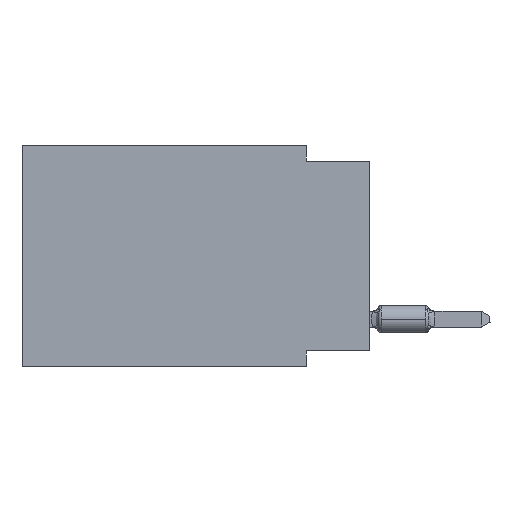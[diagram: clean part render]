
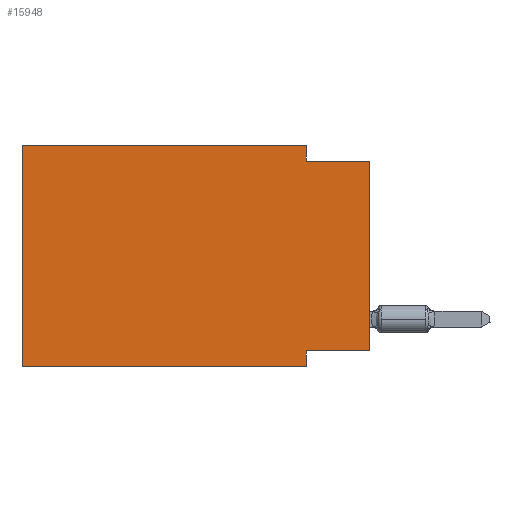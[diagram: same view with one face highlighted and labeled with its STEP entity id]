
A CAD part, left-side view. The second image highlights one B-rep face of the part: STEP entity #15948.
In plain terms, the highlighted planar face has unit normal (-1, 0, 0).
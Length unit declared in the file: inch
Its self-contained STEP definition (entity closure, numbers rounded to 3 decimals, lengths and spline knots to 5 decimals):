
#21 = VERTEX_POINT ( 'NONE', #21464 ) ;
#82 = PLANE ( 'NONE',  #12504 ) ;
#561 = ORIENTED_EDGE ( 'NONE', *, *, #11492, .F. ) ;
#1091 = DIRECTION ( 'NONE',  ( 0., -1., 0. ) ) ;
#1288 = VECTOR ( 'NONE', #1091, 39.37008 ) ;
#1444 = CARTESIAN_POINT ( 'NONE',  ( 0., 0.55, -0.35 ) ) ;
#1791 = LINE ( 'NONE', #2118, #21281 ) ;
#1793 = VECTOR ( 'NONE', #25685, 39.37008 ) ;
#2018 = CARTESIAN_POINT ( 'NONE',  ( 0., 0.1, 0. ) ) ;
#2118 = CARTESIAN_POINT ( 'NONE',  ( 0., 0., -0.325 ) ) ;
#2986 = VERTEX_POINT ( 'NONE', #25995 ) ;
#3607 = ORIENTED_EDGE ( 'NONE', *, *, #14719, .F. ) ;
#3935 = LINE ( 'NONE', #24307, #24319 ) ;
#4313 = VECTOR ( 'NONE', #11893, 39.37008 ) ;
#4394 = CARTESIAN_POINT ( 'NONE',  ( 0., 0.1, -0.35 ) ) ;
#4684 = LINE ( 'NONE', #2018, #8402 ) ;
#4748 = FACE_OUTER_BOUND ( 'NONE', #13828, .T. ) ;
#6435 = DIRECTION ( 'NONE',  ( 0., -1., 0. ) ) ;
#7199 = DIRECTION ( 'NONE',  ( 0., 0., 1. ) ) ;
#7359 = CARTESIAN_POINT ( 'NONE',  ( 0., 0.55, 0. ) ) ;
#8402 = VECTOR ( 'NONE', #19878, 39.37008 ) ;
#8758 = ORIENTED_EDGE ( 'NONE', *, *, #14175, .T. ) ;
#9121 = VERTEX_POINT ( 'NONE', #12037 ) ;
#9704 = LINE ( 'NONE', #7359, #22607 ) ;
#11492 = EDGE_CURVE ( 'NONE', #9121, #15752, #24458, .T. ) ;
#11893 = DIRECTION ( 'NONE',  ( 0., 0., -1. ) ) ;
#11947 = ORIENTED_EDGE ( 'NONE', *, *, #30300, .T. ) ;
#12037 = CARTESIAN_POINT ( 'NONE',  ( 0., 0.1, -0.025 ) ) ;
#12504 = AXIS2_PLACEMENT_3D ( 'NONE', #31055, #20281, #25122 ) ;
#13427 = CARTESIAN_POINT ( 'NONE',  ( 0., 0., -0.025 ) ) ;
#13828 = EDGE_LOOP ( 'NONE', ( #8758, #561, #17830, #32062, #3607, #11947, #24671, #23426 ) ) ;
#14175 = EDGE_CURVE ( 'NONE', #21798, #15752, #25358, .T. ) ;
#14464 = LINE ( 'NONE', #1444, #17566 ) ;
#14719 = EDGE_CURVE ( 'NONE', #21, #19742, #9704, .T. ) ;
#15066 = VERTEX_POINT ( 'NONE', #27208 ) ;
#15752 = VERTEX_POINT ( 'NONE', #13427 ) ;
#15948 = ADVANCED_FACE ( 'NONE', ( #4748 ), #82, .F. ) ;
#16985 = CARTESIAN_POINT ( 'NONE',  ( 0., 0.1, -0.35 ) ) ;
#17094 = LINE ( 'NONE', #4394, #4313 ) ;
#17566 = VECTOR ( 'NONE', #24662, 39.37008 ) ;
#17830 = ORIENTED_EDGE ( 'NONE', *, *, #28786, .F. ) ;
#19742 = VERTEX_POINT ( 'NONE', #25765 ) ;
#19813 = DIRECTION ( 'NONE',  ( 0., 1., 0. ) ) ;
#19878 = DIRECTION ( 'NONE',  ( 0., 0., -1. ) ) ;
#20281 = DIRECTION ( 'NONE',  ( 1., 0., 0. ) ) ;
#21281 = VECTOR ( 'NONE', #19813, 39.37008 ) ;
#21464 = CARTESIAN_POINT ( 'NONE',  ( 0., 0.55, -0.35 ) ) ;
#21798 = VERTEX_POINT ( 'NONE', #23988 ) ;
#21951 = EDGE_CURVE ( 'NONE', #21798, #15066, #1791, .T. ) ;
#22607 = VECTOR ( 'NONE', #7199, 39.37008 ) ;
#23426 = ORIENTED_EDGE ( 'NONE', *, *, #21951, .F. ) ;
#23745 = EDGE_CURVE ( 'NONE', #15066, #31570, #17094, .T. ) ;
#23959 = CARTESIAN_POINT ( 'NONE',  ( 0., 0., -0.025 ) ) ;
#23988 = CARTESIAN_POINT ( 'NONE',  ( 0., 0., -0.325 ) ) ;
#24307 = CARTESIAN_POINT ( 'NONE',  ( 0., 0.55, 0. ) ) ;
#24319 = VECTOR ( 'NONE', #6435, 39.37008 ) ;
#24458 = LINE ( 'NONE', #23959, #1288 ) ;
#24662 = DIRECTION ( 'NONE',  ( 0., -1., 0. ) ) ;
#24671 = ORIENTED_EDGE ( 'NONE', *, *, #23745, .F. ) ;
#24906 = EDGE_CURVE ( 'NONE', #19742, #2986, #3935, .T. ) ;
#25122 = DIRECTION ( 'NONE',  ( 0., 0., -1. ) ) ;
#25358 = LINE ( 'NONE', #30518, #1793 ) ;
#25685 = DIRECTION ( 'NONE',  ( 0., 0., 1. ) ) ;
#25765 = CARTESIAN_POINT ( 'NONE',  ( 0., 0.55, 0. ) ) ;
#25995 = CARTESIAN_POINT ( 'NONE',  ( 0., 0.1, 0. ) ) ;
#27208 = CARTESIAN_POINT ( 'NONE',  ( 0., 0.1, -0.325 ) ) ;
#28786 = EDGE_CURVE ( 'NONE', #2986, #9121, #4684, .T. ) ;
#30300 = EDGE_CURVE ( 'NONE', #21, #31570, #14464, .T. ) ;
#30518 = CARTESIAN_POINT ( 'NONE',  ( 0., 0., 0. ) ) ;
#31055 = CARTESIAN_POINT ( 'NONE',  ( 0., 0.55, 0. ) ) ;
#31570 = VERTEX_POINT ( 'NONE', #16985 ) ;
#32062 = ORIENTED_EDGE ( 'NONE', *, *, #24906, .F. ) ;
